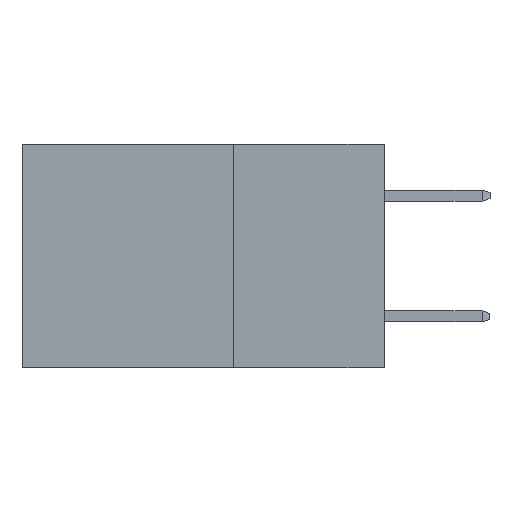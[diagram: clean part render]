
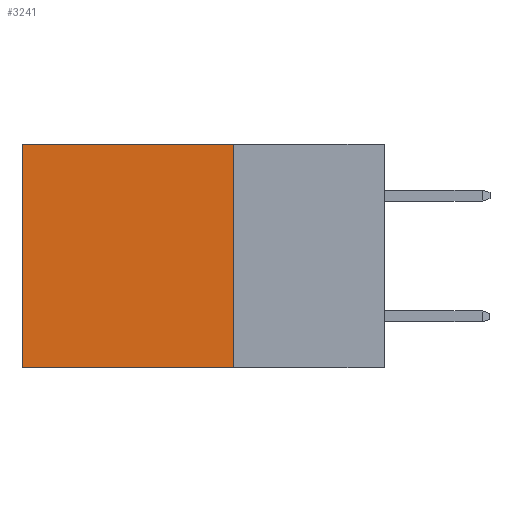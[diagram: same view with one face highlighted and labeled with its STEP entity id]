
A CAD part, left-side view. The second image highlights one B-rep face of the part: STEP entity #3241.
In plain terms, the highlighted planar face has unit normal (-1, 0, 0).
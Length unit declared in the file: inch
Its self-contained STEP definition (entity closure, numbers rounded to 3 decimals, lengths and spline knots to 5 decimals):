
#162 = CARTESIAN_POINT ( 'NONE',  ( 0.298, 0.25, 0. ) ) ;
#329 = VERTEX_POINT ( 'NONE', #5616 ) ;
#411 = EDGE_CURVE ( 'NONE', #2251, #329, #12728, .T. ) ;
#693 = EDGE_CURVE ( 'NONE', #11680, #10726, #5108, .T. ) ;
#2251 = VERTEX_POINT ( 'NONE', #12488 ) ;
#2515 = DIRECTION ( 'NONE',  ( 0., 0., -1. ) ) ;
#3241 = ADVANCED_FACE ( 'NONE', ( #5988 ), #13198, .F. ) ;
#3441 = DIRECTION ( 'NONE',  ( 1., 0., 0. ) ) ;
#3580 = VECTOR ( 'NONE', #9906, 39.37008 ) ;
#3836 = DIRECTION ( 'NONE',  ( 0., 1., 0. ) ) ;
#4080 = EDGE_CURVE ( 'NONE', #10726, #329, #11243, .T. ) ;
#4319 = DIRECTION ( 'NONE',  ( 0., 0., -1. ) ) ;
#4388 = ORIENTED_EDGE ( 'NONE', *, *, #411, .F. ) ;
#4536 = CARTESIAN_POINT ( 'NONE',  ( 0.298, 0.25, 0. ) ) ;
#5108 = LINE ( 'NONE', #10852, #11375 ) ;
#5199 = ORIENTED_EDGE ( 'NONE', *, *, #4080, .T. ) ;
#5616 = CARTESIAN_POINT ( 'NONE',  ( 0.298, 0.6, -0.37 ) ) ;
#5988 = FACE_OUTER_BOUND ( 'NONE', #12107, .T. ) ;
#7502 = VECTOR ( 'NONE', #4319, 39.37008 ) ;
#7732 = CARTESIAN_POINT ( 'NONE',  ( 0.298, 0.25, 0. ) ) ;
#8721 = ORIENTED_EDGE ( 'NONE', *, *, #10250, .F. ) ;
#9796 = ORIENTED_EDGE ( 'NONE', *, *, #693, .T. ) ;
#9906 = DIRECTION ( 'NONE',  ( 0., 0., -1. ) ) ;
#9926 = DIRECTION ( 'NONE',  ( 0., 1., 0. ) ) ;
#10250 = EDGE_CURVE ( 'NONE', #11680, #2251, #11369, .T. ) ;
#10390 = AXIS2_PLACEMENT_3D ( 'NONE', #4536, #3441, #2515 ) ;
#10726 = VERTEX_POINT ( 'NONE', #14500 ) ;
#10787 = CARTESIAN_POINT ( 'NONE',  ( 0.298, 0.6, 0. ) ) ;
#10852 = CARTESIAN_POINT ( 'NONE',  ( 0.298, 0.25, 0. ) ) ;
#11243 = LINE ( 'NONE', #10787, #7502 ) ;
#11369 = LINE ( 'NONE', #162, #3580 ) ;
#11375 = VECTOR ( 'NONE', #3836, 39.37008 ) ;
#11680 = VERTEX_POINT ( 'NONE', #7732 ) ;
#12107 = EDGE_LOOP ( 'NONE', ( #5199, #4388, #8721, #9796 ) ) ;
#12355 = VECTOR ( 'NONE', #9926, 39.37008 ) ;
#12488 = CARTESIAN_POINT ( 'NONE',  ( 0.298, 0.25, -0.37 ) ) ;
#12728 = LINE ( 'NONE', #13351, #12355 ) ;
#13198 = PLANE ( 'NONE',  #10390 ) ;
#13351 = CARTESIAN_POINT ( 'NONE',  ( 0.298, 0.25, -0.37 ) ) ;
#14500 = CARTESIAN_POINT ( 'NONE',  ( 0.298, 0.6, 0. ) ) ;
